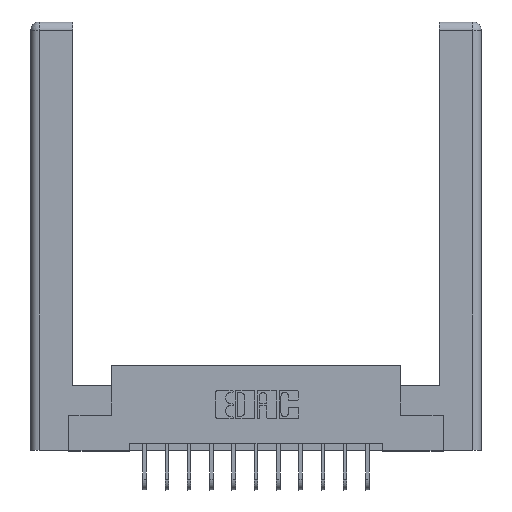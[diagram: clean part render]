
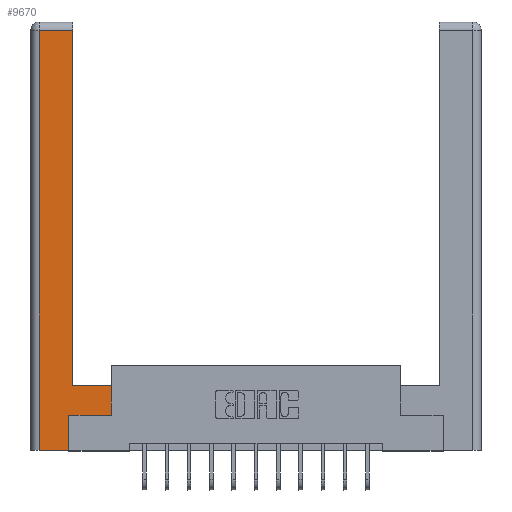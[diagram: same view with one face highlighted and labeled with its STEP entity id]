
A CAD part, top view. The second image highlights one B-rep face of the part: STEP entity #9670.
In plain terms, the highlighted planar face has unit normal (0, 0, 1).
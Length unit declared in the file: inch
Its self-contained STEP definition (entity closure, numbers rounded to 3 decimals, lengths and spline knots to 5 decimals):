
#220 = CARTESIAN_POINT ( 'NONE',  ( 0.0615, 0., 0. ) ) ;
#550 = ORIENTED_EDGE ( 'NONE', *, *, #7164, .T. ) ;
#791 = PLANE ( 'NONE',  #11780 ) ;
#1282 = VERTEX_POINT ( 'NONE', #15839 ) ;
#1334 = CARTESIAN_POINT ( 'NONE',  ( 0.565, 0.245, 0. ) ) ;
#1493 = ORIENTED_EDGE ( 'NONE', *, *, #13441, .T. ) ;
#1775 = CARTESIAN_POINT ( 'NONE',  ( 0.295, 2.94, 0. ) ) ;
#2021 = LINE ( 'NONE', #16910, #11651 ) ;
#2331 = CARTESIAN_POINT ( 'NONE',  ( 0.265, 0., 0. ) ) ;
#2682 = LINE ( 'NONE', #3403, #5991 ) ;
#2833 = VERTEX_POINT ( 'NONE', #8898 ) ;
#3164 = EDGE_CURVE ( 'NONE', #11841, #7326, #3710, .T. ) ;
#3403 = CARTESIAN_POINT ( 'NONE',  ( 0.565, 0.245, 0. ) ) ;
#3566 = ORIENTED_EDGE ( 'NONE', *, *, #13794, .T. ) ;
#3593 = ORIENTED_EDGE ( 'NONE', *, *, #11431, .T. ) ;
#3710 = LINE ( 'NONE', #9558, #12538 ) ;
#3762 = CARTESIAN_POINT ( 'NONE',  ( 0.565, 0.45, 0. ) ) ;
#3875 = LINE ( 'NONE', #4295, #11484 ) ;
#4227 = VECTOR ( 'NONE', #6847, 39.37008 ) ;
#4295 = CARTESIAN_POINT ( 'NONE',  ( 0.295, 3., 0. ) ) ;
#4363 = DIRECTION ( 'NONE',  ( 0., 1., 0. ) ) ;
#5764 = VERTEX_POINT ( 'NONE', #220 ) ;
#5991 = VECTOR ( 'NONE', #12686, 39.37008 ) ;
#6152 = VECTOR ( 'NONE', #12259, 39.37008 ) ;
#6524 = VECTOR ( 'NONE', #12534, 39.37008 ) ;
#6539 = DIRECTION ( 'NONE',  ( -1., 0., 0. ) ) ;
#6824 = DIRECTION ( 'NONE',  ( 0., 1., 0. ) ) ;
#6847 = DIRECTION ( 'NONE',  ( 0., -1., 0. ) ) ;
#7081 = DIRECTION ( 'NONE',  ( -1., 0., 0. ) ) ;
#7164 = EDGE_CURVE ( 'NONE', #2833, #10032, #10424, .T. ) ;
#7258 = CARTESIAN_POINT ( 'NONE',  ( 0.0615, 2.94, 0. ) ) ;
#7308 = EDGE_LOOP ( 'NONE', ( #9373, #10471, #3566, #1493, #550, #9775, #16441, #3593 ) ) ;
#7326 = VERTEX_POINT ( 'NONE', #3762 ) ;
#7482 = CARTESIAN_POINT ( 'NONE',  ( 0., 0., 0. ) ) ;
#7973 = VECTOR ( 'NONE', #7081, 39.37008 ) ;
#8540 = CARTESIAN_POINT ( 'NONE',  ( 0.265, 0.245, 0. ) ) ;
#8898 = CARTESIAN_POINT ( 'NONE',  ( 0.265, 0., 0. ) ) ;
#9373 = ORIENTED_EDGE ( 'NONE', *, *, #10957, .T. ) ;
#9558 = CARTESIAN_POINT ( 'NONE',  ( 0.565, 0.45, 0. ) ) ;
#9670 = ADVANCED_FACE ( 'NONE', ( #11938 ), #791, .F. ) ;
#9775 = ORIENTED_EDGE ( 'NONE', *, *, #16705, .T. ) ;
#10032 = VERTEX_POINT ( 'NONE', #8540 ) ;
#10424 = LINE ( 'NONE', #13967, #6152 ) ;
#10471 = ORIENTED_EDGE ( 'NONE', *, *, #12693, .T. ) ;
#10668 = VERTEX_POINT ( 'NONE', #1775 ) ;
#10953 = CARTESIAN_POINT ( 'NONE',  ( 0.295, 0.45, 0. ) ) ;
#10957 = EDGE_CURVE ( 'NONE', #1282, #10668, #3875, .T. ) ;
#11215 = LINE ( 'NONE', #12047, #4227 ) ;
#11431 = EDGE_CURVE ( 'NONE', #7326, #1282, #15929, .T. ) ;
#11479 = DIRECTION ( 'NONE',  ( 0., 0., -1. ) ) ;
#11484 = VECTOR ( 'NONE', #4363, 39.37008 ) ;
#11651 = VECTOR ( 'NONE', #6539, 39.37008 ) ;
#11780 = AXIS2_PLACEMENT_3D ( 'NONE', #7482, #11479, #13804 ) ;
#11841 = VERTEX_POINT ( 'NONE', #1334 ) ;
#11938 = FACE_OUTER_BOUND ( 'NONE', #7308, .T. ) ;
#12047 = CARTESIAN_POINT ( 'NONE',  ( 0.0615, 0., 0. ) ) ;
#12259 = DIRECTION ( 'NONE',  ( 0., 1., 0. ) ) ;
#12534 = DIRECTION ( 'NONE',  ( 1., 0., 0. ) ) ;
#12538 = VECTOR ( 'NONE', #6824, 39.37008 ) ;
#12686 = DIRECTION ( 'NONE',  ( 1., 0., 0. ) ) ;
#12693 = EDGE_CURVE ( 'NONE', #10668, #14724, #2021, .T. ) ;
#13441 = EDGE_CURVE ( 'NONE', #5764, #2833, #13461, .T. ) ;
#13461 = LINE ( 'NONE', #2331, #6524 ) ;
#13794 = EDGE_CURVE ( 'NONE', #14724, #5764, #11215, .T. ) ;
#13804 = DIRECTION ( 'NONE',  ( -1., 0., 0. ) ) ;
#13967 = CARTESIAN_POINT ( 'NONE',  ( 0.265, 0.245, 0. ) ) ;
#14724 = VERTEX_POINT ( 'NONE', #7258 ) ;
#15839 = CARTESIAN_POINT ( 'NONE',  ( 0.295, 0.45, 0. ) ) ;
#15929 = LINE ( 'NONE', #10953, #7973 ) ;
#16441 = ORIENTED_EDGE ( 'NONE', *, *, #3164, .T. ) ;
#16705 = EDGE_CURVE ( 'NONE', #10032, #11841, #2682, .T. ) ;
#16910 = CARTESIAN_POINT ( 'NONE',  ( 0.0615, 2.94, 0. ) ) ;
